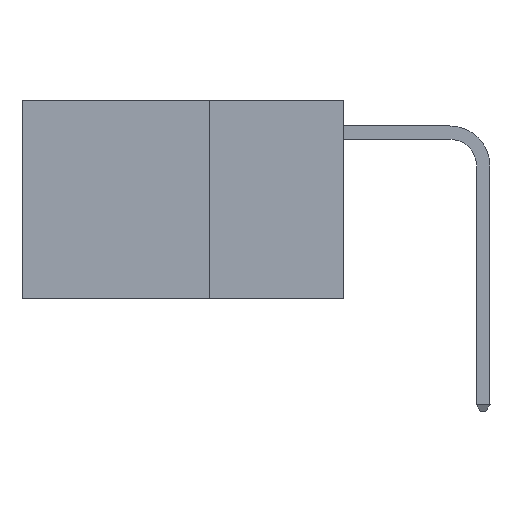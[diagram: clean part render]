
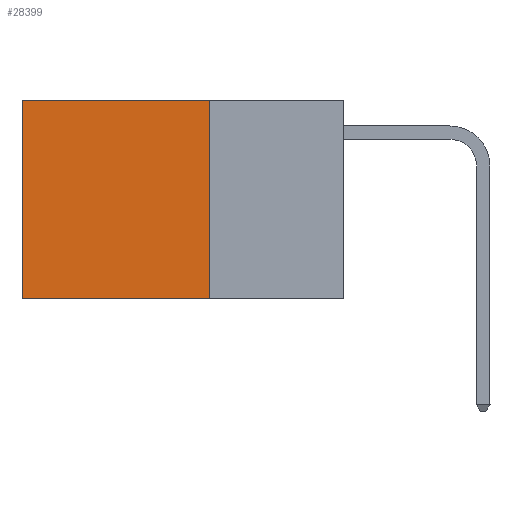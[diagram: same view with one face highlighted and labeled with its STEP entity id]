
A CAD part, left-side view. The second image highlights one B-rep face of the part: STEP entity #28399.
In plain terms, the highlighted planar face has unit normal (-1, 0, 0).
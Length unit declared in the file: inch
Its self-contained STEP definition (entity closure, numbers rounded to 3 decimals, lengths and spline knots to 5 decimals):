
#104 = CARTESIAN_POINT ( 'NONE',  ( 0.2625, 0.25, 0. ) ) ;
#1736 = EDGE_CURVE ( 'NONE', #8483, #4461, #26801, .T. ) ;
#2393 = DIRECTION ( 'NONE',  ( 0., 0., -1. ) ) ;
#3111 = LINE ( 'NONE', #10247, #14536 ) ;
#3183 = ORIENTED_EDGE ( 'NONE', *, *, #23719, .F. ) ;
#3681 = CARTESIAN_POINT ( 'NONE',  ( 0.2625, 0.25, 0. ) ) ;
#4461 = VERTEX_POINT ( 'NONE', #16115 ) ;
#4628 = EDGE_CURVE ( 'NONE', #27347, #19837, #3111, .T. ) ;
#4891 = ORIENTED_EDGE ( 'NONE', *, *, #18552, .T. ) ;
#5109 = DIRECTION ( 'NONE',  ( 1., 0., 0. ) ) ;
#7739 = CARTESIAN_POINT ( 'NONE',  ( 0.2625, 0.25, 0. ) ) ;
#8483 = VERTEX_POINT ( 'NONE', #3681 ) ;
#9042 = ORIENTED_EDGE ( 'NONE', *, *, #1736, .T. ) ;
#9550 = VECTOR ( 'NONE', #23544, 39.37008 ) ;
#10013 = CARTESIAN_POINT ( 'NONE',  ( 0.2625, 0.25, -0.37 ) ) ;
#10247 = CARTESIAN_POINT ( 'NONE',  ( 0.2625, 0.25, -0.37 ) ) ;
#10408 = CARTESIAN_POINT ( 'NONE',  ( 0.2625, 0.6, 0. ) ) ;
#14480 = AXIS2_PLACEMENT_3D ( 'NONE', #18704, #5109, #20951 ) ;
#14536 = VECTOR ( 'NONE', #28252, 39.37008 ) ;
#14785 = ORIENTED_EDGE ( 'NONE', *, *, #4628, .F. ) ;
#14815 = CARTESIAN_POINT ( 'NONE',  ( 0.2625, 0.6, -0.37 ) ) ;
#15992 = VECTOR ( 'NONE', #2393, 39.37008 ) ;
#16115 = CARTESIAN_POINT ( 'NONE',  ( 0.2625, 0.6, 0. ) ) ;
#16719 = LINE ( 'NONE', #104, #15992 ) ;
#18105 = LINE ( 'NONE', #10408, #29267 ) ;
#18552 = EDGE_CURVE ( 'NONE', #4461, #19837, #18105, .T. ) ;
#18704 = CARTESIAN_POINT ( 'NONE',  ( 0.2625, 0.25, 0. ) ) ;
#19837 = VERTEX_POINT ( 'NONE', #14815 ) ;
#20951 = DIRECTION ( 'NONE',  ( 0., 0., -1. ) ) ;
#23544 = DIRECTION ( 'NONE',  ( 0., 1., 0. ) ) ;
#23719 = EDGE_CURVE ( 'NONE', #8483, #27347, #16719, .T. ) ;
#24067 = FACE_OUTER_BOUND ( 'NONE', #27237, .T. ) ;
#25318 = PLANE ( 'NONE',  #14480 ) ;
#26801 = LINE ( 'NONE', #7739, #9550 ) ;
#27237 = EDGE_LOOP ( 'NONE', ( #4891, #14785, #3183, #9042 ) ) ;
#27347 = VERTEX_POINT ( 'NONE', #10013 ) ;
#28252 = DIRECTION ( 'NONE',  ( 0., 1., 0. ) ) ;
#28399 = ADVANCED_FACE ( 'NONE', ( #24067 ), #25318, .F. ) ;
#28413 = DIRECTION ( 'NONE',  ( 0., 0., -1. ) ) ;
#29267 = VECTOR ( 'NONE', #28413, 39.37008 ) ;
